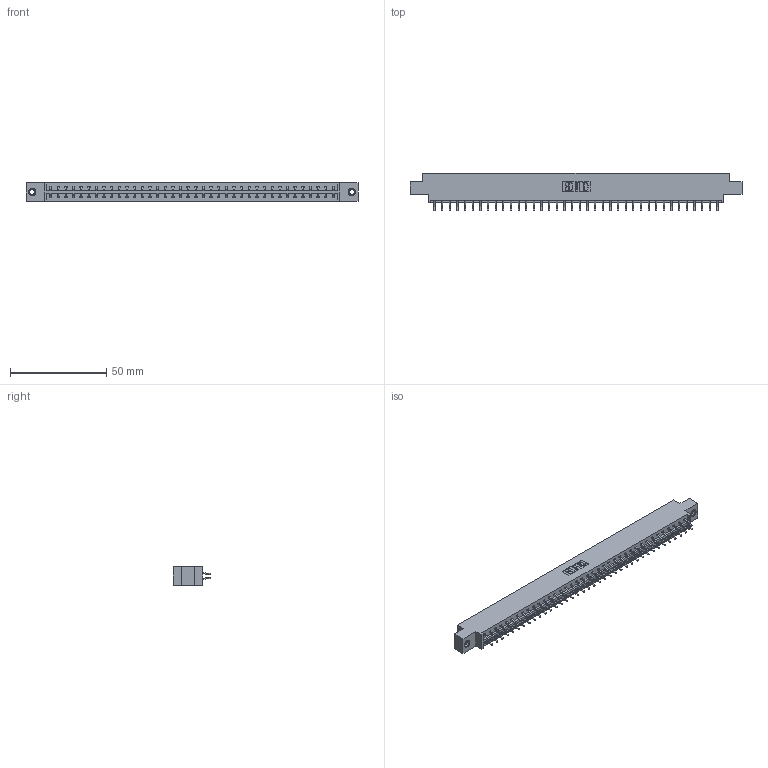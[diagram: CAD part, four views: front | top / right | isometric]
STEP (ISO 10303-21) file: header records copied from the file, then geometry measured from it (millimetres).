
FILE_DESCRIPTION (( 'STEP AP203' ), '1' );
FILE_NAME ('833-076-556-807.STEP', '2020-06-05T18:57:40', ( '' ), ( '' ), 'SwSTEP 2.0', 'SolidWorks 2020', '' );
FILE_SCHEMA (( 'CONFIG_CONTROL_DESIGN' ));
Length unit declared in the file: inch
Products named in the file (4): 345-250-001_345-250-005-103; 833-076-556-807; 345-292-001_556 Tail; 833 Part_Offset - .156 Dia - TI
Assembly tree (79 placements, depth 2):
  833-076-556-807
    833 Part_Offset - .156 Dia - TI
    345-292-001_556 Tail  x76
    345-250-001_345-250-005-103  x2
Bounding box: 172.11 x 19.57 x 9.4 mm (x, y, z)
Volume: 17289.8 mm3; surface area: 20577.8 mm2
Topology: 79 solids, 79 shells, 4586 faces, 13607 edges, 8962 vertices
Faces by surface type: plane 3146, cylinder 1424, cone 12, torus 4
Entity records: 26502 total; most frequent: CARTESIAN_POINT 4397, ORIENTED_EDGE 4314, DIRECTION 3783, EDGE_CURVE 2157, LINE 2001, VECTOR 2001, VERTEX_POINT 1432, AXIS2_PLACEMENT_3D 891
